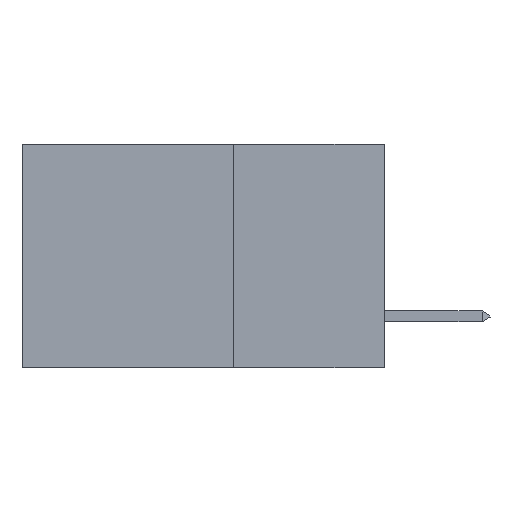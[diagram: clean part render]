
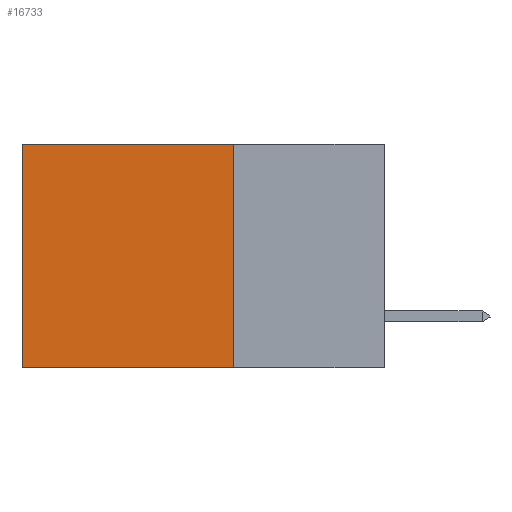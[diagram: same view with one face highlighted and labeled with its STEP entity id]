
A CAD part, left-side view. The second image highlights one B-rep face of the part: STEP entity #16733.
In plain terms, the highlighted planar face has unit normal (-1, 0, 0).
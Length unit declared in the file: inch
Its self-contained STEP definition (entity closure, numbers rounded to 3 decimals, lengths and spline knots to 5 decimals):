
#1091 = PLANE ( 'NONE',  #4355 ) ;
#1268 = EDGE_CURVE ( 'NONE', #15655, #5533, #9959, .T. ) ;
#1363 = ORIENTED_EDGE ( 'NONE', *, *, #4646, .F. ) ;
#2191 = EDGE_CURVE ( 'NONE', #15655, #6877, #9534, .T. ) ;
#2506 = DIRECTION ( 'NONE',  ( 0., 1., 0. ) ) ;
#4355 = AXIS2_PLACEMENT_3D ( 'NONE', #13973, #5949, #8975 ) ;
#4646 = EDGE_CURVE ( 'NONE', #6877, #12190, #20578, .T. ) ;
#5533 = VERTEX_POINT ( 'NONE', #17462 ) ;
#5833 = ORIENTED_EDGE ( 'NONE', *, *, #6093, .T. ) ;
#5949 = DIRECTION ( 'NONE',  ( 1., 0., 0. ) ) ;
#6093 = EDGE_CURVE ( 'NONE', #5533, #12190, #8111, .T. ) ;
#6877 = VERTEX_POINT ( 'NONE', #17460 ) ;
#7378 = CARTESIAN_POINT ( 'NONE',  ( 0.2875, 0.25, 0. ) ) ;
#7953 = DIRECTION ( 'NONE',  ( 0., 0., -1. ) ) ;
#8111 = LINE ( 'NONE', #15284, #9379 ) ;
#8372 = CARTESIAN_POINT ( 'NONE',  ( 0.2875, 0.6, -0.37 ) ) ;
#8465 = VECTOR ( 'NONE', #2506, 39.37008 ) ;
#8537 = EDGE_LOOP ( 'NONE', ( #5833, #1363, #18220, #15375 ) ) ;
#8975 = DIRECTION ( 'NONE',  ( 0., 0., -1. ) ) ;
#9379 = VECTOR ( 'NONE', #7953, 39.37008 ) ;
#9534 = LINE ( 'NONE', #16695, #20210 ) ;
#9792 = CARTESIAN_POINT ( 'NONE',  ( 0.2875, 0.25, -0.37 ) ) ;
#9959 = LINE ( 'NONE', #7378, #8465 ) ;
#10440 = FACE_OUTER_BOUND ( 'NONE', #8537, .T. ) ;
#12190 = VERTEX_POINT ( 'NONE', #8372 ) ;
#13973 = CARTESIAN_POINT ( 'NONE',  ( 0.2875, 0.25, 0. ) ) ;
#15028 = DIRECTION ( 'NONE',  ( 0., 0., -1. ) ) ;
#15065 = DIRECTION ( 'NONE',  ( 0., 1., 0. ) ) ;
#15284 = CARTESIAN_POINT ( 'NONE',  ( 0.2875, 0.6, 0. ) ) ;
#15375 = ORIENTED_EDGE ( 'NONE', *, *, #1268, .T. ) ;
#15655 = VERTEX_POINT ( 'NONE', #19385 ) ;
#16427 = VECTOR ( 'NONE', #15065, 39.37008 ) ;
#16695 = CARTESIAN_POINT ( 'NONE',  ( 0.2875, 0.25, 0. ) ) ;
#16733 = ADVANCED_FACE ( 'NONE', ( #10440 ), #1091, .F. ) ;
#17460 = CARTESIAN_POINT ( 'NONE',  ( 0.2875, 0.25, -0.37 ) ) ;
#17462 = CARTESIAN_POINT ( 'NONE',  ( 0.2875, 0.6, 0. ) ) ;
#18220 = ORIENTED_EDGE ( 'NONE', *, *, #2191, .F. ) ;
#19385 = CARTESIAN_POINT ( 'NONE',  ( 0.2875, 0.25, 0. ) ) ;
#20210 = VECTOR ( 'NONE', #15028, 39.37008 ) ;
#20578 = LINE ( 'NONE', #9792, #16427 ) ;
